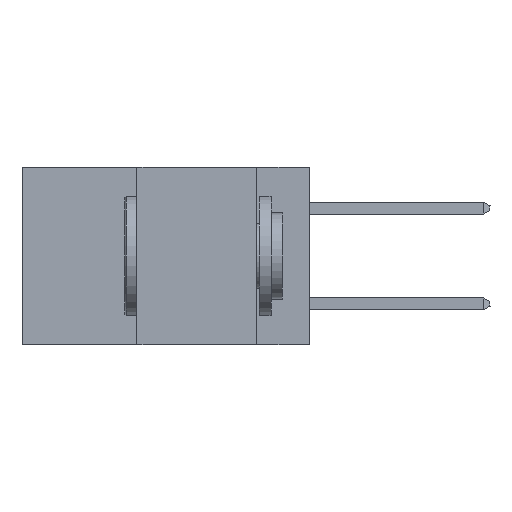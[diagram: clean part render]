
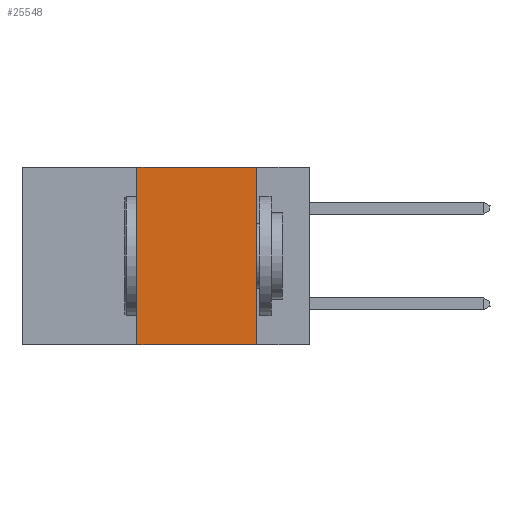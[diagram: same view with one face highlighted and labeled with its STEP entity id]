
A CAD part, left-side view. The second image highlights one B-rep face of the part: STEP entity #25548.
In plain terms, the highlighted planar face has unit normal (-1, 0, 0).
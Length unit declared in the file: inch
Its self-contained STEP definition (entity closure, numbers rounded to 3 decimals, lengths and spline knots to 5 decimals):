
#91 = EDGE_LOOP ( 'NONE', ( #8538, #43047, #28613, #1578 ) ) ;
#1496 = FACE_OUTER_BOUND ( 'NONE', #91, .T. ) ;
#1578 = ORIENTED_EDGE ( 'NONE', *, *, #32223, .T. ) ;
#2797 = DIRECTION ( 'NONE',  ( 1., 0., 0. ) ) ;
#4155 = VERTEX_POINT ( 'NONE', #39948 ) ;
#4321 = CARTESIAN_POINT ( 'NONE',  ( 0., 0.11, 0. ) ) ;
#5783 = DIRECTION ( 'NONE',  ( 0., 0., -1. ) ) ;
#7078 = CARTESIAN_POINT ( 'NONE',  ( 0., 0.36, 0. ) ) ;
#8538 = ORIENTED_EDGE ( 'NONE', *, *, #11796, .F. ) ;
#9888 = CARTESIAN_POINT ( 'NONE',  ( 0., 0.11, 0. ) ) ;
#10208 = LINE ( 'NONE', #19982, #12358 ) ;
#11796 = EDGE_CURVE ( 'NONE', #39214, #38932, #23218, .T. ) ;
#12189 = VECTOR ( 'NONE', #15676, 39.37008 ) ;
#12358 = VECTOR ( 'NONE', #29824, 39.37008 ) ;
#13654 = VERTEX_POINT ( 'NONE', #22214 ) ;
#14106 = VECTOR ( 'NONE', #31695, 39.37008 ) ;
#15676 = DIRECTION ( 'NONE',  ( 0., -1., 0. ) ) ;
#19982 = CARTESIAN_POINT ( 'NONE',  ( 0., 0.6, 0. ) ) ;
#20605 = LINE ( 'NONE', #7078, #34448 ) ;
#22214 = CARTESIAN_POINT ( 'NONE',  ( 0., 0.36, 0. ) ) ;
#23218 = LINE ( 'NONE', #4321, #14106 ) ;
#25548 = ADVANCED_FACE ( 'NONE', ( #1496 ), #39795, .F. ) ;
#25859 = EDGE_CURVE ( 'NONE', #4155, #13654, #20605, .T. ) ;
#25986 = AXIS2_PLACEMENT_3D ( 'NONE', #29444, #2797, #5783 ) ;
#28613 = ORIENTED_EDGE ( 'NONE', *, *, #25859, .F. ) ;
#29444 = CARTESIAN_POINT ( 'NONE',  ( 0., 0.6, 0. ) ) ;
#29824 = DIRECTION ( 'NONE',  ( 0., -1., 0. ) ) ;
#30644 = EDGE_CURVE ( 'NONE', #13654, #39214, #10208, .T. ) ;
#31695 = DIRECTION ( 'NONE',  ( 0., 0., -1. ) ) ;
#32223 = EDGE_CURVE ( 'NONE', #4155, #38932, #35124, .T. ) ;
#34448 = VECTOR ( 'NONE', #37802, 39.37008 ) ;
#35124 = LINE ( 'NONE', #36111, #12189 ) ;
#36111 = CARTESIAN_POINT ( 'NONE',  ( 0., 0.6, -0.37 ) ) ;
#37802 = DIRECTION ( 'NONE',  ( 0., 0., 1. ) ) ;
#38932 = VERTEX_POINT ( 'NONE', #42014 ) ;
#39214 = VERTEX_POINT ( 'NONE', #9888 ) ;
#39795 = PLANE ( 'NONE',  #25986 ) ;
#39948 = CARTESIAN_POINT ( 'NONE',  ( 0., 0.36, -0.37 ) ) ;
#42014 = CARTESIAN_POINT ( 'NONE',  ( 0., 0.11, -0.37 ) ) ;
#43047 = ORIENTED_EDGE ( 'NONE', *, *, #30644, .F. ) ;
